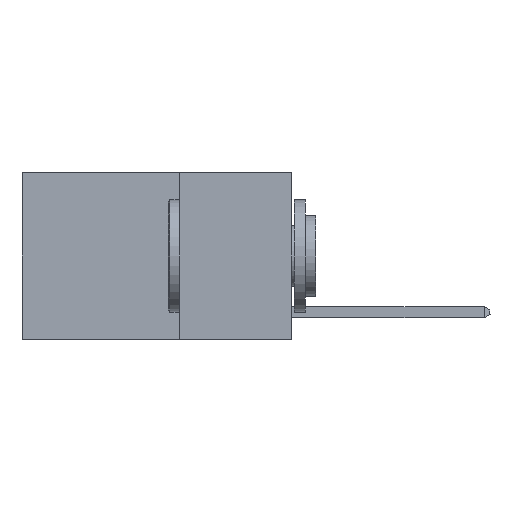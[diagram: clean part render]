
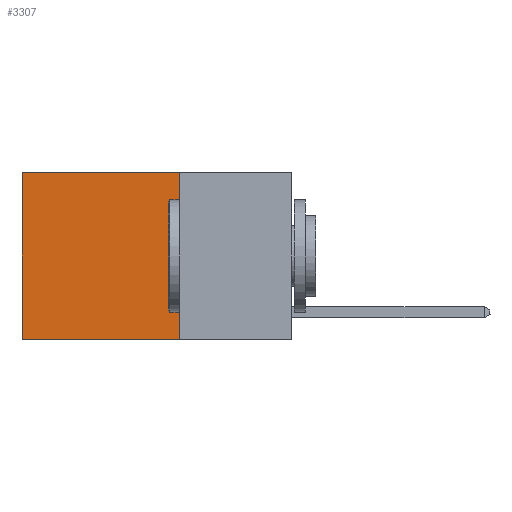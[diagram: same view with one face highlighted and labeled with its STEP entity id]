
A CAD part, left-side view. The second image highlights one B-rep face of the part: STEP entity #3307.
In plain terms, the highlighted planar face has unit normal (-1, 0, 0).
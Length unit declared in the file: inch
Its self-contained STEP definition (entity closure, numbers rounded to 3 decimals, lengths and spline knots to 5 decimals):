
#260 = CARTESIAN_POINT ( 'NONE',  ( 0.2625, 0.25, 0. ) ) ;
#261 = CARTESIAN_POINT ( 'NONE',  ( 0.2625, 0.6, 0. ) ) ;
#384 = LINE ( 'NONE', #6737, #1304 ) ;
#854 = EDGE_CURVE ( 'NONE', #2772, #3627, #384, .T. ) ;
#1304 = VECTOR ( 'NONE', #5382, 39.37008 ) ;
#1718 = ORIENTED_EDGE ( 'NONE', *, *, #6284, .T. ) ;
#1782 = DIRECTION ( 'NONE',  ( 0., 0., -1. ) ) ;
#2453 = LINE ( 'NONE', #3834, #3847 ) ;
#2772 = VERTEX_POINT ( 'NONE', #7225 ) ;
#2816 = ORIENTED_EDGE ( 'NONE', *, *, #3368, .F. ) ;
#3307 = ADVANCED_FACE ( 'NONE', ( #4552 ), #8855, .F. ) ;
#3368 = EDGE_CURVE ( 'NONE', #7721, #2772, #5863, .T. ) ;
#3625 = CARTESIAN_POINT ( 'NONE',  ( 0.2625, 0.25, 0. ) ) ;
#3627 = VERTEX_POINT ( 'NONE', #8041 ) ;
#3737 = EDGE_CURVE ( 'NONE', #7721, #8140, #2453, .T. ) ;
#3834 = CARTESIAN_POINT ( 'NONE',  ( 0.2625, 0.25, 0. ) ) ;
#3847 = VECTOR ( 'NONE', #8240, 39.37008 ) ;
#4551 = LINE ( 'NONE', #5250, #5445 ) ;
#4552 = FACE_OUTER_BOUND ( 'NONE', #5982, .T. ) ;
#4607 = DIRECTION ( 'NONE',  ( 0., 0., -1. ) ) ;
#5250 = CARTESIAN_POINT ( 'NONE',  ( 0.2625, 0.6, 0. ) ) ;
#5382 = DIRECTION ( 'NONE',  ( 0., 1., 0. ) ) ;
#5445 = VECTOR ( 'NONE', #1782, 39.37008 ) ;
#5494 = AXIS2_PLACEMENT_3D ( 'NONE', #6703, #8811, #4607 ) ;
#5776 = VECTOR ( 'NONE', #5955, 39.37008 ) ;
#5863 = LINE ( 'NONE', #260, #5776 ) ;
#5955 = DIRECTION ( 'NONE',  ( 0., 0., -1. ) ) ;
#5982 = EDGE_LOOP ( 'NONE', ( #1718, #8528, #2816, #6211 ) ) ;
#6211 = ORIENTED_EDGE ( 'NONE', *, *, #3737, .T. ) ;
#6284 = EDGE_CURVE ( 'NONE', #8140, #3627, #4551, .T. ) ;
#6703 = CARTESIAN_POINT ( 'NONE',  ( 0.2625, 0.25, 0. ) ) ;
#6737 = CARTESIAN_POINT ( 'NONE',  ( 0.2625, 0.25, -0.37 ) ) ;
#7225 = CARTESIAN_POINT ( 'NONE',  ( 0.2625, 0.25, -0.37 ) ) ;
#7721 = VERTEX_POINT ( 'NONE', #3625 ) ;
#8041 = CARTESIAN_POINT ( 'NONE',  ( 0.2625, 0.6, -0.37 ) ) ;
#8140 = VERTEX_POINT ( 'NONE', #261 ) ;
#8240 = DIRECTION ( 'NONE',  ( 0., 1., 0. ) ) ;
#8528 = ORIENTED_EDGE ( 'NONE', *, *, #854, .F. ) ;
#8811 = DIRECTION ( 'NONE',  ( 1., 0., 0. ) ) ;
#8855 = PLANE ( 'NONE',  #5494 ) ;
